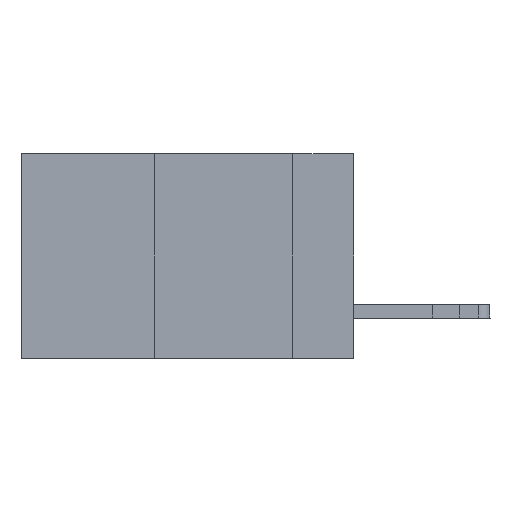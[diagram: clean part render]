
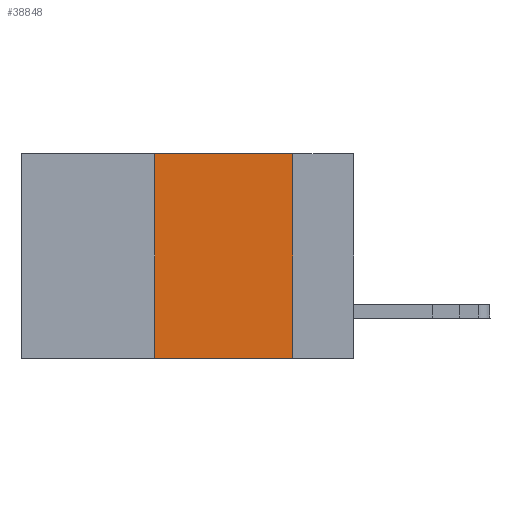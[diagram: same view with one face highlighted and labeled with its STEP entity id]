
A CAD part, left-side view. The second image highlights one B-rep face of the part: STEP entity #38848.
In plain terms, the highlighted planar face has unit normal (-1, 0, 0).
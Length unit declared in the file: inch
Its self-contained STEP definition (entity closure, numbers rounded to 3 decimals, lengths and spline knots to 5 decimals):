
#3329 = VECTOR ( 'NONE', #5301, 39.37008 ) ;
#3731 = ORIENTED_EDGE ( 'NONE', *, *, #24965, .T. ) ;
#5301 = DIRECTION ( 'NONE',  ( 0., 0., -1. ) ) ;
#7466 = DIRECTION ( 'NONE',  ( 0., -1., 0. ) ) ;
#8258 = LINE ( 'NONE', #29419, #3329 ) ;
#8483 = CARTESIAN_POINT ( 'NONE',  ( 0., 0.11, -0.37 ) ) ;
#8498 = EDGE_CURVE ( 'NONE', #12813, #38246, #10414, .T. ) ;
#9127 = DIRECTION ( 'NONE',  ( 0., 0., 1. ) ) ;
#10414 = LINE ( 'NONE', #15949, #17359 ) ;
#11146 = AXIS2_PLACEMENT_3D ( 'NONE', #32908, #29929, #14880 ) ;
#11926 = FACE_OUTER_BOUND ( 'NONE', #36518, .T. ) ;
#12080 = EDGE_CURVE ( 'NONE', #20898, #12813, #24165, .T. ) ;
#12333 = CARTESIAN_POINT ( 'NONE',  ( 0., 0.36, -0.37 ) ) ;
#12813 = VERTEX_POINT ( 'NONE', #33564 ) ;
#14880 = DIRECTION ( 'NONE',  ( 0., 0., -1. ) ) ;
#15949 = CARTESIAN_POINT ( 'NONE',  ( 0., 0.6, 0. ) ) ;
#16476 = VECTOR ( 'NONE', #35644, 39.37008 ) ;
#16752 = ORIENTED_EDGE ( 'NONE', *, *, #34498, .F. ) ;
#16906 = CARTESIAN_POINT ( 'NONE',  ( 0., 0.11, 0. ) ) ;
#17359 = VECTOR ( 'NONE', #7466, 39.37008 ) ;
#18653 = VERTEX_POINT ( 'NONE', #8483 ) ;
#20898 = VERTEX_POINT ( 'NONE', #12333 ) ;
#23198 = VECTOR ( 'NONE', #9127, 39.37008 ) ;
#23989 = PLANE ( 'NONE',  #11146 ) ;
#24144 = CARTESIAN_POINT ( 'NONE',  ( 0., 0.6, -0.37 ) ) ;
#24165 = LINE ( 'NONE', #26939, #23198 ) ;
#24965 = EDGE_CURVE ( 'NONE', #20898, #18653, #35841, .T. ) ;
#26939 = CARTESIAN_POINT ( 'NONE',  ( 0., 0.36, 0. ) ) ;
#29419 = CARTESIAN_POINT ( 'NONE',  ( 0., 0.11, 0. ) ) ;
#29929 = DIRECTION ( 'NONE',  ( 1., 0., 0. ) ) ;
#30784 = ORIENTED_EDGE ( 'NONE', *, *, #8498, .F. ) ;
#32267 = ORIENTED_EDGE ( 'NONE', *, *, #12080, .F. ) ;
#32908 = CARTESIAN_POINT ( 'NONE',  ( 0., 0.6, 0. ) ) ;
#33564 = CARTESIAN_POINT ( 'NONE',  ( 0., 0.36, 0. ) ) ;
#34498 = EDGE_CURVE ( 'NONE', #38246, #18653, #8258, .T. ) ;
#35644 = DIRECTION ( 'NONE',  ( 0., -1., 0. ) ) ;
#35841 = LINE ( 'NONE', #24144, #16476 ) ;
#36518 = EDGE_LOOP ( 'NONE', ( #16752, #30784, #32267, #3731 ) ) ;
#38246 = VERTEX_POINT ( 'NONE', #16906 ) ;
#38848 = ADVANCED_FACE ( 'NONE', ( #11926 ), #23989, .F. ) ;
